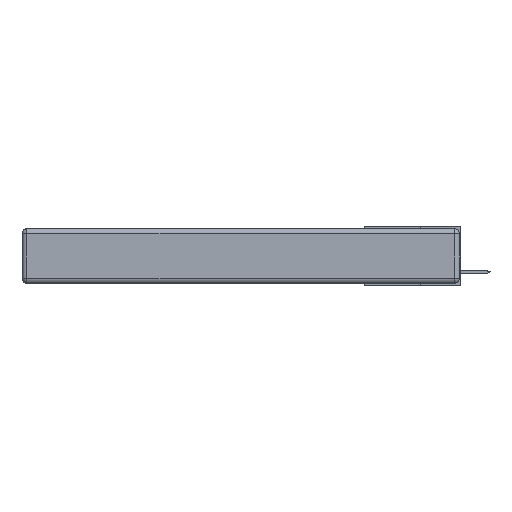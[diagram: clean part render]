
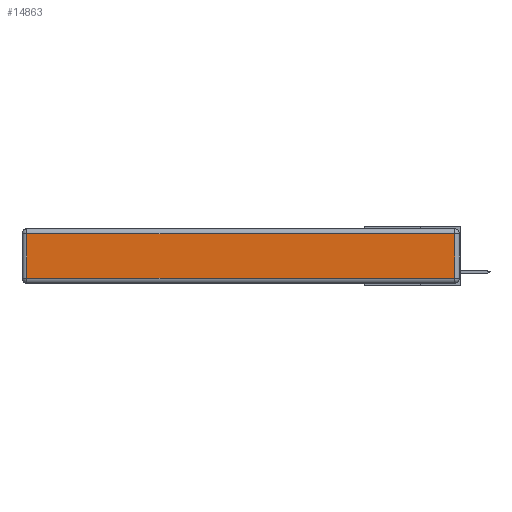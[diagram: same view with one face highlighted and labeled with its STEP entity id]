
A CAD part, left-side view. The second image highlights one B-rep face of the part: STEP entity #14863.
In plain terms, the highlighted planar face has unit normal (-1, 0, 0).
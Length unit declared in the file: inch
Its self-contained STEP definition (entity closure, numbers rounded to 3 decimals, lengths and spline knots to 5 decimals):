
#147 = EDGE_CURVE ( 'NONE', #25113, #19918, #4979, .T. ) ;
#1816 = LINE ( 'NONE', #6757, #5585 ) ;
#2324 = CARTESIAN_POINT ( 'NONE',  ( 0., 2.72, -0.03 ) ) ;
#2629 = CARTESIAN_POINT ( 'NONE',  ( 0., 0.03, -0.03 ) ) ;
#3048 = CARTESIAN_POINT ( 'NONE',  ( 0., 0.03, -0.343 ) ) ;
#3676 = VECTOR ( 'NONE', #7590, 39.37008 ) ;
#4699 = DIRECTION ( 'NONE',  ( 0., 0., 1. ) ) ;
#4809 = CARTESIAN_POINT ( 'NONE',  ( 0., 0.03, -0.313 ) ) ;
#4979 = LINE ( 'NONE', #13292, #22919 ) ;
#5585 = VECTOR ( 'NONE', #13254, 39.37008 ) ;
#6757 = CARTESIAN_POINT ( 'NONE',  ( 0., 0., -0.313 ) ) ;
#7590 = DIRECTION ( 'NONE',  ( 0., 0., 1. ) ) ;
#8081 = VECTOR ( 'NONE', #16595, 39.37008 ) ;
#8802 = CARTESIAN_POINT ( 'NONE',  ( 0., 0., -0.343 ) ) ;
#8928 = EDGE_CURVE ( 'NONE', #19918, #14745, #1816, .T. ) ;
#9293 = ORIENTED_EDGE ( 'NONE', *, *, #8928, .T. ) ;
#11457 = ORIENTED_EDGE ( 'NONE', *, *, #147, .T. ) ;
#13254 = DIRECTION ( 'NONE',  ( 0., -1., 0. ) ) ;
#13292 = CARTESIAN_POINT ( 'NONE',  ( 0., 2.72, -0.343 ) ) ;
#14745 = VERTEX_POINT ( 'NONE', #4809 ) ;
#14863 = ADVANCED_FACE ( 'NONE', ( #19668 ), #22183, .T. ) ;
#15746 = EDGE_CURVE ( 'NONE', #14745, #16149, #24752, .T. ) ;
#16085 = LINE ( 'NONE', #27235, #8081 ) ;
#16149 = VERTEX_POINT ( 'NONE', #2629 ) ;
#16518 = ORIENTED_EDGE ( 'NONE', *, *, #21942, .T. ) ;
#16595 = DIRECTION ( 'NONE',  ( 0., 1., 0. ) ) ;
#17957 = DIRECTION ( 'NONE',  ( -1., 0., 0. ) ) ;
#19055 = AXIS2_PLACEMENT_3D ( 'NONE', #8802, #17957, #4699 ) ;
#19668 = FACE_OUTER_BOUND ( 'NONE', #26909, .T. ) ;
#19918 = VERTEX_POINT ( 'NONE', #26462 ) ;
#21942 = EDGE_CURVE ( 'NONE', #16149, #25113, #16085, .T. ) ;
#22183 = PLANE ( 'NONE',  #19055 ) ;
#22919 = VECTOR ( 'NONE', #28348, 39.37008 ) ;
#24752 = LINE ( 'NONE', #3048, #3676 ) ;
#25113 = VERTEX_POINT ( 'NONE', #2324 ) ;
#25169 = ORIENTED_EDGE ( 'NONE', *, *, #15746, .T. ) ;
#26462 = CARTESIAN_POINT ( 'NONE',  ( 0., 2.72, -0.313 ) ) ;
#26909 = EDGE_LOOP ( 'NONE', ( #9293, #25169, #16518, #11457 ) ) ;
#27235 = CARTESIAN_POINT ( 'NONE',  ( 0., 2.75, -0.03 ) ) ;
#28348 = DIRECTION ( 'NONE',  ( 0., 0., -1. ) ) ;
